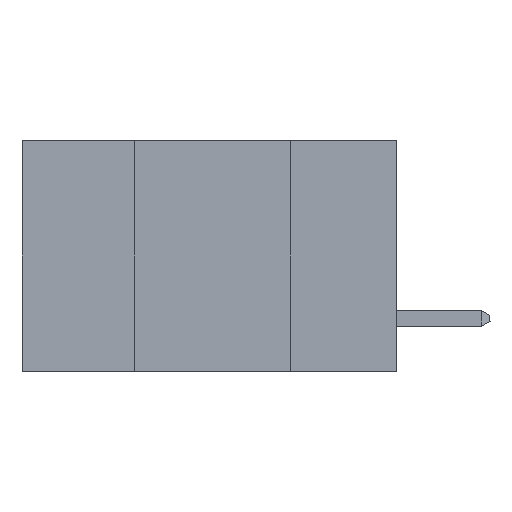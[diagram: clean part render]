
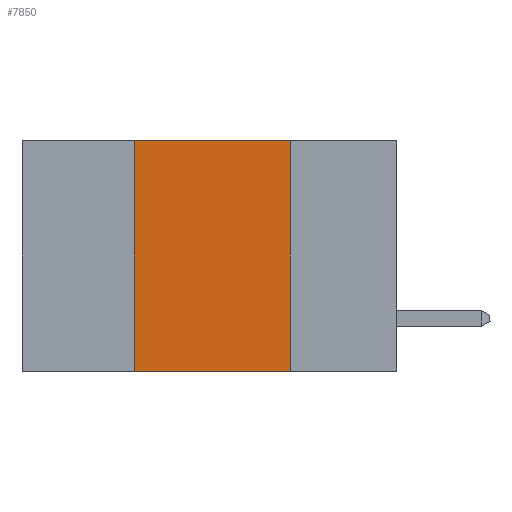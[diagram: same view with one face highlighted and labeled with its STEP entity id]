
A CAD part, left-side view. The second image highlights one B-rep face of the part: STEP entity #7850.
In plain terms, the highlighted planar face has unit normal (-1, 0, 0).
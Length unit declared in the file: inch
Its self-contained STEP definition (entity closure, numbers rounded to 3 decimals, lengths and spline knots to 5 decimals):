
#436 = VERTEX_POINT ( 'NONE', #13375 ) ;
#502 = CARTESIAN_POINT ( 'NONE',  ( 0., 0.17, 0. ) ) ;
#538 = AXIS2_PLACEMENT_3D ( 'NONE', #11267, #4558, #12358 ) ;
#888 = ORIENTED_EDGE ( 'NONE', *, *, #10569, .F. ) ;
#1627 = VERTEX_POINT ( 'NONE', #6323 ) ;
#2999 = DIRECTION ( 'NONE',  ( 0., 0., -1. ) ) ;
#3333 = PLANE ( 'NONE',  #538 ) ;
#3364 = CARTESIAN_POINT ( 'NONE',  ( 0., 0.17, -0.37 ) ) ;
#3529 = DIRECTION ( 'NONE',  ( 0., -1., 0. ) ) ;
#3710 = VERTEX_POINT ( 'NONE', #7711 ) ;
#4549 = ORIENTED_EDGE ( 'NONE', *, *, #6041, .T. ) ;
#4558 = DIRECTION ( 'NONE',  ( 1., 0., 0. ) ) ;
#4834 = FACE_OUTER_BOUND ( 'NONE', #8014, .T. ) ;
#6041 = EDGE_CURVE ( 'NONE', #436, #12372, #6844, .T. ) ;
#6323 = CARTESIAN_POINT ( 'NONE',  ( 0., 0.17, 0. ) ) ;
#6370 = CARTESIAN_POINT ( 'NONE',  ( 0., 0.6, -0.37 ) ) ;
#6750 = EDGE_CURVE ( 'NONE', #3710, #1627, #7862, .T. ) ;
#6844 = LINE ( 'NONE', #6370, #9485 ) ;
#6856 = ORIENTED_EDGE ( 'NONE', *, *, #6750, .F. ) ;
#7253 = VECTOR ( 'NONE', #2999, 39.37008 ) ;
#7467 = LINE ( 'NONE', #12171, #12946 ) ;
#7711 = CARTESIAN_POINT ( 'NONE',  ( 0., 0.42, 0. ) ) ;
#7850 = ADVANCED_FACE ( 'NONE', ( #4834 ), #3333, .F. ) ;
#7862 = LINE ( 'NONE', #12519, #8213 ) ;
#8014 = EDGE_LOOP ( 'NONE', ( #888, #6856, #10531, #4549 ) ) ;
#8213 = VECTOR ( 'NONE', #3529, 39.37008 ) ;
#9092 = EDGE_CURVE ( 'NONE', #436, #3710, #7467, .T. ) ;
#9485 = VECTOR ( 'NONE', #12492, 39.37008 ) ;
#10531 = ORIENTED_EDGE ( 'NONE', *, *, #9092, .F. ) ;
#10569 = EDGE_CURVE ( 'NONE', #1627, #12372, #10572, .T. ) ;
#10572 = LINE ( 'NONE', #502, #7253 ) ;
#11267 = CARTESIAN_POINT ( 'NONE',  ( 0., 0.6, 0. ) ) ;
#12171 = CARTESIAN_POINT ( 'NONE',  ( 0., 0.42, 0. ) ) ;
#12358 = DIRECTION ( 'NONE',  ( 0., 0., -1. ) ) ;
#12372 = VERTEX_POINT ( 'NONE', #3364 ) ;
#12492 = DIRECTION ( 'NONE',  ( 0., -1., 0. ) ) ;
#12519 = CARTESIAN_POINT ( 'NONE',  ( 0., 0.6, 0. ) ) ;
#12946 = VECTOR ( 'NONE', #13245, 39.37008 ) ;
#13245 = DIRECTION ( 'NONE',  ( 0., 0., 1. ) ) ;
#13375 = CARTESIAN_POINT ( 'NONE',  ( 0., 0.42, -0.37 ) ) ;
